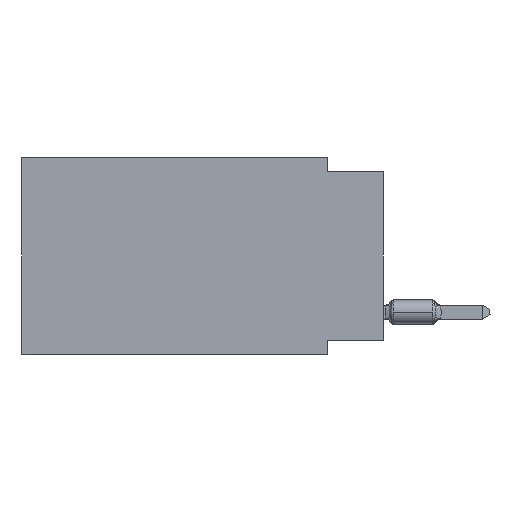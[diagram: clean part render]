
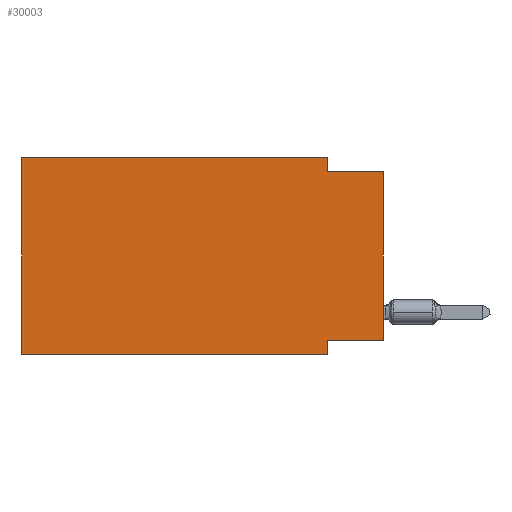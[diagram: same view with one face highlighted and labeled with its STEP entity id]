
A CAD part, left-side view. The second image highlights one B-rep face of the part: STEP entity #30003.
In plain terms, the highlighted planar face has unit normal (-1, 0, 0).
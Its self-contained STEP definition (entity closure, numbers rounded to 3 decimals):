
#596 = CARTESIAN_POINT ( 'NONE',  ( 0., 0., -8.255 ) ) ;
#633 = ORIENTED_EDGE ( 'NONE', *, *, #18953, .T. ) ;
#1053 = EDGE_CURVE ( 'NONE', #6079, #8301, #31136, .T. ) ;
#1314 = VECTOR ( 'NONE', #30623, 1000. ) ;
#1794 = CARTESIAN_POINT ( 'NONE',  ( 0., 2.54, -0.635 ) ) ;
#3370 = VERTEX_POINT ( 'NONE', #1794 ) ;
#3495 = CARTESIAN_POINT ( 'NONE',  ( 0., 2.54, -8.89 ) ) ;
#3906 = ORIENTED_EDGE ( 'NONE', *, *, #14746, .F. ) ;
#4437 = LINE ( 'NONE', #34676, #30134 ) ;
#6079 = VERTEX_POINT ( 'NONE', #12134 ) ;
#8301 = VERTEX_POINT ( 'NONE', #21060 ) ;
#9372 = AXIS2_PLACEMENT_3D ( 'NONE', #32555, #32751, #11013 ) ;
#9611 = CARTESIAN_POINT ( 'NONE',  ( 0., 0., 0. ) ) ;
#9940 = DIRECTION ( 'NONE',  ( 0., 0., 1. ) ) ;
#10135 = CARTESIAN_POINT ( 'NONE',  ( 0., 16.383, 0. ) ) ;
#10507 = LINE ( 'NONE', #13299, #21961 ) ;
#10931 = VECTOR ( 'NONE', #24830, 1000. ) ;
#11013 = DIRECTION ( 'NONE',  ( 0., 0., -1. ) ) ;
#11588 = EDGE_CURVE ( 'NONE', #6079, #23438, #13421, .T. ) ;
#11807 = VECTOR ( 'NONE', #32459, 1000. ) ;
#12134 = CARTESIAN_POINT ( 'NONE',  ( 0., 0., -8.255 ) ) ;
#13176 = VECTOR ( 'NONE', #27674, 1000. ) ;
#13241 = CARTESIAN_POINT ( 'NONE',  ( 0., 2.54, 0. ) ) ;
#13299 = CARTESIAN_POINT ( 'NONE',  ( 0., 16.383, 0. ) ) ;
#13421 = LINE ( 'NONE', #596, #13176 ) ;
#14746 = EDGE_CURVE ( 'NONE', #24833, #3370, #21545, .T. ) ;
#15163 = LINE ( 'NONE', #32545, #18753 ) ;
#15429 = CARTESIAN_POINT ( 'NONE',  ( 0., 2.54, 0. ) ) ;
#18029 = CARTESIAN_POINT ( 'NONE',  ( 0., 2.54, -8.89 ) ) ;
#18753 = VECTOR ( 'NONE', #38466, 1000. ) ;
#18843 = ORIENTED_EDGE ( 'NONE', *, *, #34423, .F. ) ;
#18953 = EDGE_CURVE ( 'NONE', #24364, #38146, #23162, .T. ) ;
#19178 = EDGE_LOOP ( 'NONE', ( #32419, #28689, #3906, #25836, #30511, #633, #18843, #28595 ) ) ;
#19776 = EDGE_CURVE ( 'NONE', #24364, #27927, #10507, .T. ) ;
#20801 = LINE ( 'NONE', #18029, #24625 ) ;
#21060 = CARTESIAN_POINT ( 'NONE',  ( 0., 0., -0.635 ) ) ;
#21545 = LINE ( 'NONE', #15429, #1314 ) ;
#21961 = VECTOR ( 'NONE', #9940, 1000. ) ;
#23162 = LINE ( 'NONE', #29478, #11807 ) ;
#23438 = VERTEX_POINT ( 'NONE', #31943 ) ;
#23596 = EDGE_CURVE ( 'NONE', #27927, #24833, #15163, .T. ) ;
#24364 = VERTEX_POINT ( 'NONE', #24967 ) ;
#24625 = VECTOR ( 'NONE', #35212, 1000. ) ;
#24830 = DIRECTION ( 'NONE',  ( 0., 0., 1. ) ) ;
#24833 = VERTEX_POINT ( 'NONE', #13241 ) ;
#24967 = CARTESIAN_POINT ( 'NONE',  ( 0., 16.383, -8.89 ) ) ;
#25836 = ORIENTED_EDGE ( 'NONE', *, *, #23596, .F. ) ;
#27674 = DIRECTION ( 'NONE',  ( 0., 1., 0. ) ) ;
#27806 = DIRECTION ( 'NONE',  ( 0., -1., 0. ) ) ;
#27927 = VERTEX_POINT ( 'NONE', #10135 ) ;
#28595 = ORIENTED_EDGE ( 'NONE', *, *, #11588, .F. ) ;
#28689 = ORIENTED_EDGE ( 'NONE', *, *, #30406, .F. ) ;
#29001 = PLANE ( 'NONE',  #9372 ) ;
#29478 = CARTESIAN_POINT ( 'NONE',  ( 0., 16.383, -8.89 ) ) ;
#29796 = FACE_OUTER_BOUND ( 'NONE', #19178, .T. ) ;
#30003 = ADVANCED_FACE ( 'NONE', ( #29796 ), #29001, .F. ) ;
#30134 = VECTOR ( 'NONE', #27806, 1000. ) ;
#30406 = EDGE_CURVE ( 'NONE', #3370, #8301, #4437, .T. ) ;
#30511 = ORIENTED_EDGE ( 'NONE', *, *, #19776, .F. ) ;
#30623 = DIRECTION ( 'NONE',  ( 0., 0., -1. ) ) ;
#31136 = LINE ( 'NONE', #9611, #10931 ) ;
#31943 = CARTESIAN_POINT ( 'NONE',  ( 0., 2.54, -8.255 ) ) ;
#32419 = ORIENTED_EDGE ( 'NONE', *, *, #1053, .T. ) ;
#32459 = DIRECTION ( 'NONE',  ( 0., -1., 0. ) ) ;
#32545 = CARTESIAN_POINT ( 'NONE',  ( 0., 16.383, 0. ) ) ;
#32555 = CARTESIAN_POINT ( 'NONE',  ( 0., 16.383, 0. ) ) ;
#32751 = DIRECTION ( 'NONE',  ( 1., 0., 0. ) ) ;
#34423 = EDGE_CURVE ( 'NONE', #23438, #38146, #20801, .T. ) ;
#34676 = CARTESIAN_POINT ( 'NONE',  ( 0., 0., -0.635 ) ) ;
#35212 = DIRECTION ( 'NONE',  ( 0., 0., -1. ) ) ;
#38146 = VERTEX_POINT ( 'NONE', #3495 ) ;
#38466 = DIRECTION ( 'NONE',  ( 0., -1., 0. ) ) ;
